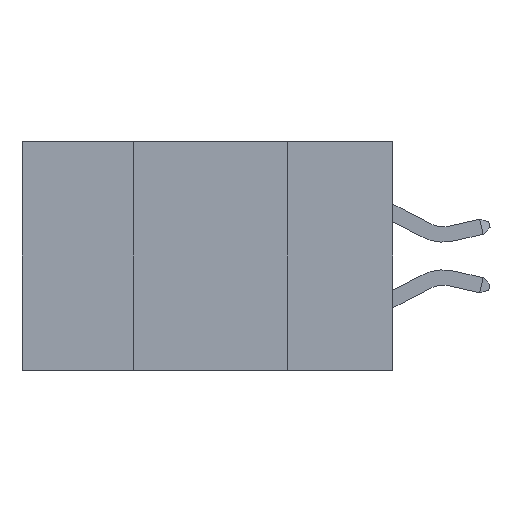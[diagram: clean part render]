
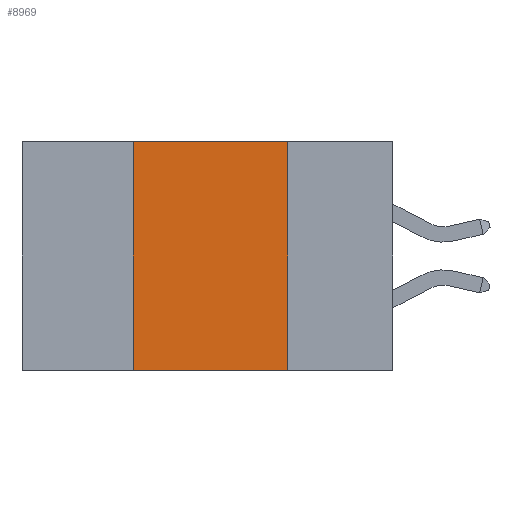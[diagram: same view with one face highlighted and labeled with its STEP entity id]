
A CAD part, left-side view. The second image highlights one B-rep face of the part: STEP entity #8969.
In plain terms, the highlighted planar face has unit normal (-1, 0, 0).
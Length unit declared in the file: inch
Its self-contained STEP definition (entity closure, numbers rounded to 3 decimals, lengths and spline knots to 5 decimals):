
#520 = EDGE_CURVE ( 'NONE', #16402, #9237, #17079, .T. ) ;
#842 = CARTESIAN_POINT ( 'NONE',  ( 0., 0.42, 0. ) ) ;
#1456 = VECTOR ( 'NONE', #8227, 39.37008 ) ;
#1983 = FACE_OUTER_BOUND ( 'NONE', #8148, .T. ) ;
#3464 = DIRECTION ( 'NONE',  ( 1., 0., 0. ) ) ;
#4504 = EDGE_CURVE ( 'NONE', #9237, #14394, #13581, .T. ) ;
#4943 = PLANE ( 'NONE',  #14546 ) ;
#5251 = CARTESIAN_POINT ( 'NONE',  ( 0., 0.6, -0.37 ) ) ;
#5523 = CARTESIAN_POINT ( 'NONE',  ( 0., 0.6, 0. ) ) ;
#5564 = LINE ( 'NONE', #842, #1456 ) ;
#6094 = CARTESIAN_POINT ( 'NONE',  ( 0., 0.17, 0. ) ) ;
#6455 = ORIENTED_EDGE ( 'NONE', *, *, #520, .F. ) ;
#8148 = EDGE_LOOP ( 'NONE', ( #13924, #6455, #15744, #18703 ) ) ;
#8227 = DIRECTION ( 'NONE',  ( 0., 0., 1. ) ) ;
#8388 = VECTOR ( 'NONE', #15887, 39.37008 ) ;
#8884 = VERTEX_POINT ( 'NONE', #17951 ) ;
#8969 = ADVANCED_FACE ( 'NONE', ( #1983 ), #4943, .F. ) ;
#9237 = VERTEX_POINT ( 'NONE', #9870 ) ;
#9289 = CARTESIAN_POINT ( 'NONE',  ( 0., 0.42, 0. ) ) ;
#9580 = CARTESIAN_POINT ( 'NONE',  ( 0., 0.6, 0. ) ) ;
#9870 = CARTESIAN_POINT ( 'NONE',  ( 0., 0.17, 0. ) ) ;
#10061 = DIRECTION ( 'NONE',  ( 0., -1., 0. ) ) ;
#11260 = VECTOR ( 'NONE', #12094, 39.37008 ) ;
#11536 = VECTOR ( 'NONE', #10061, 39.37008 ) ;
#12094 = DIRECTION ( 'NONE',  ( 0., 0., -1. ) ) ;
#13581 = LINE ( 'NONE', #6094, #11260 ) ;
#13924 = ORIENTED_EDGE ( 'NONE', *, *, #4504, .F. ) ;
#14394 = VERTEX_POINT ( 'NONE', #15053 ) ;
#14546 = AXIS2_PLACEMENT_3D ( 'NONE', #9580, #3464, #15589 ) ;
#15053 = CARTESIAN_POINT ( 'NONE',  ( 0., 0.17, -0.37 ) ) ;
#15589 = DIRECTION ( 'NONE',  ( 0., 0., -1. ) ) ;
#15744 = ORIENTED_EDGE ( 'NONE', *, *, #16171, .F. ) ;
#15887 = DIRECTION ( 'NONE',  ( 0., -1., 0. ) ) ;
#16171 = EDGE_CURVE ( 'NONE', #8884, #16402, #5564, .T. ) ;
#16402 = VERTEX_POINT ( 'NONE', #9289 ) ;
#16607 = EDGE_CURVE ( 'NONE', #8884, #14394, #17359, .T. ) ;
#17079 = LINE ( 'NONE', #5523, #11536 ) ;
#17359 = LINE ( 'NONE', #5251, #8388 ) ;
#17951 = CARTESIAN_POINT ( 'NONE',  ( 0., 0.42, -0.37 ) ) ;
#18703 = ORIENTED_EDGE ( 'NONE', *, *, #16607, .T. ) ;
